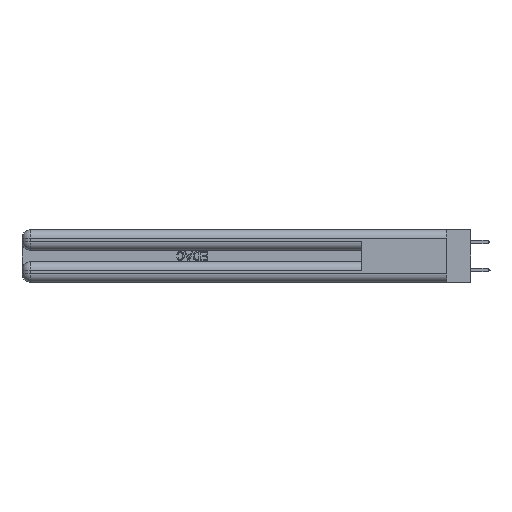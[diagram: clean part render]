
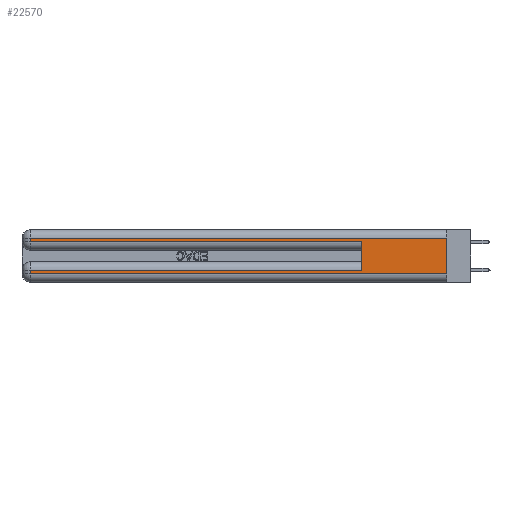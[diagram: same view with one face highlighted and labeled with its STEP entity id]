
A CAD part, left-side view. The second image highlights one B-rep face of the part: STEP entity #22570.
In plain terms, the highlighted planar face has unit normal (-1, 0, 0).
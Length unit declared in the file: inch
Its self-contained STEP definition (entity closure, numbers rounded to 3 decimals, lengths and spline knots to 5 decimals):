
#603 = VERTEX_POINT ( 'NONE', #787 ) ;
#787 = CARTESIAN_POINT ( 'NONE',  ( 0., 0., 0.06 ) ) ;
#1549 = CARTESIAN_POINT ( 'NONE',  ( 0., 0.6, 0.085 ) ) ;
#2010 = ORIENTED_EDGE ( 'NONE', *, *, #20438, .T. ) ;
#2688 = AXIS2_PLACEMENT_3D ( 'NONE', #24120, #33008, #30104 ) ;
#3725 = PLANE ( 'NONE',  #2688 ) ;
#4019 = ORIENTED_EDGE ( 'NONE', *, *, #25882, .T. ) ;
#4820 = CARTESIAN_POINT ( 'NONE',  ( 0., 2.94, 0.285 ) ) ;
#5132 = VECTOR ( 'NONE', #10139, 39.37008 ) ;
#6074 = VERTEX_POINT ( 'NONE', #20393 ) ;
#6150 = VECTOR ( 'NONE', #32973, 39.37008 ) ;
#6956 = ORIENTED_EDGE ( 'NONE', *, *, #29617, .F. ) ;
#9332 = DIRECTION ( 'NONE',  ( 0., 1., 0. ) ) ;
#9511 = DIRECTION ( 'NONE',  ( 0., -1., 0. ) ) ;
#10139 = DIRECTION ( 'NONE',  ( 0., 0., -1. ) ) ;
#10300 = DIRECTION ( 'NONE',  ( 0., 0., -1. ) ) ;
#11101 = VECTOR ( 'NONE', #22137, 39.37008 ) ;
#11802 = CARTESIAN_POINT ( 'NONE',  ( 0., 0., 0.31 ) ) ;
#13338 = LINE ( 'NONE', #15310, #22964 ) ;
#13473 = CARTESIAN_POINT ( 'NONE',  ( 0., 2.94, 0.37 ) ) ;
#13716 = VERTEX_POINT ( 'NONE', #4820 ) ;
#14093 = CARTESIAN_POINT ( 'NONE',  ( 0., 0.6, 0.145 ) ) ;
#14237 = VECTOR ( 'NONE', #9511, 39.37008 ) ;
#15114 = ORIENTED_EDGE ( 'NONE', *, *, #32104, .T. ) ;
#15251 = DIRECTION ( 'NONE',  ( 0., -1., 0. ) ) ;
#15310 = CARTESIAN_POINT ( 'NONE',  ( 0., 0., 0.085 ) ) ;
#16123 = VECTOR ( 'NONE', #10300, 39.37008 ) ;
#16550 = VERTEX_POINT ( 'NONE', #11802 ) ;
#18145 = VERTEX_POINT ( 'NONE', #27687 ) ;
#18828 = LINE ( 'NONE', #33318, #5132 ) ;
#18955 = LINE ( 'NONE', #14093, #19896 ) ;
#19732 = ORIENTED_EDGE ( 'NONE', *, *, #25781, .T. ) ;
#19896 = VECTOR ( 'NONE', #28675, 39.37008 ) ;
#20393 = CARTESIAN_POINT ( 'NONE',  ( 0., 0.6, 0.285 ) ) ;
#20438 = EDGE_CURVE ( 'NONE', #13716, #6074, #25209, .T. ) ;
#20996 = CARTESIAN_POINT ( 'NONE',  ( 0., 0., 0.285 ) ) ;
#21740 = EDGE_CURVE ( 'NONE', #16550, #603, #18828, .T. ) ;
#22137 = DIRECTION ( 'NONE',  ( 0., 1., 0. ) ) ;
#22570 = ADVANCED_FACE ( 'NONE', ( #28123 ), #3725, .F. ) ;
#22964 = VECTOR ( 'NONE', #9332, 39.37008 ) ;
#24120 = CARTESIAN_POINT ( 'NONE',  ( 0., 0., 0.37 ) ) ;
#24797 = LINE ( 'NONE', #13473, #16123 ) ;
#25209 = LINE ( 'NONE', #20996, #14237 ) ;
#25306 = ORIENTED_EDGE ( 'NONE', *, *, #27283, .T. ) ;
#25764 = LINE ( 'NONE', #29709, #6150 ) ;
#25781 = EDGE_CURVE ( 'NONE', #33086, #33995, #25764, .T. ) ;
#25882 = EDGE_CURVE ( 'NONE', #16550, #18145, #37492, .T. ) ;
#27055 = EDGE_CURVE ( 'NONE', #28791, #33086, #13338, .T. ) ;
#27283 = EDGE_CURVE ( 'NONE', #18145, #13716, #24797, .T. ) ;
#27687 = CARTESIAN_POINT ( 'NONE',  ( 0., 2.94, 0.31 ) ) ;
#27910 = LINE ( 'NONE', #32703, #30161 ) ;
#28123 = FACE_OUTER_BOUND ( 'NONE', #31440, .T. ) ;
#28675 = DIRECTION ( 'NONE',  ( 0., 0., 1. ) ) ;
#28791 = VERTEX_POINT ( 'NONE', #1549 ) ;
#28924 = CARTESIAN_POINT ( 'NONE',  ( 0., 2.94, 0.06 ) ) ;
#29185 = ORIENTED_EDGE ( 'NONE', *, *, #27055, .T. ) ;
#29617 = EDGE_CURVE ( 'NONE', #28791, #6074, #18955, .T. ) ;
#29709 = CARTESIAN_POINT ( 'NONE',  ( 0., 2.94, 0.37 ) ) ;
#30104 = DIRECTION ( 'NONE',  ( 0., 0., -1. ) ) ;
#30161 = VECTOR ( 'NONE', #15251, 39.37008 ) ;
#31374 = CARTESIAN_POINT ( 'NONE',  ( 0., 2.94, 0.085 ) ) ;
#31440 = EDGE_LOOP ( 'NONE', ( #33961, #4019, #25306, #2010, #6956, #29185, #19732, #15114 ) ) ;
#32104 = EDGE_CURVE ( 'NONE', #33995, #603, #27910, .T. ) ;
#32703 = CARTESIAN_POINT ( 'NONE',  ( 0., 0., 0.06 ) ) ;
#32973 = DIRECTION ( 'NONE',  ( 0., 0., -1. ) ) ;
#33008 = DIRECTION ( 'NONE',  ( 1., 0., 0. ) ) ;
#33086 = VERTEX_POINT ( 'NONE', #31374 ) ;
#33318 = CARTESIAN_POINT ( 'NONE',  ( 0., 0., 0.37 ) ) ;
#33961 = ORIENTED_EDGE ( 'NONE', *, *, #21740, .F. ) ;
#33995 = VERTEX_POINT ( 'NONE', #28924 ) ;
#36349 = CARTESIAN_POINT ( 'NONE',  ( 0., 0., 0.31 ) ) ;
#37492 = LINE ( 'NONE', #36349, #11101 ) ;
